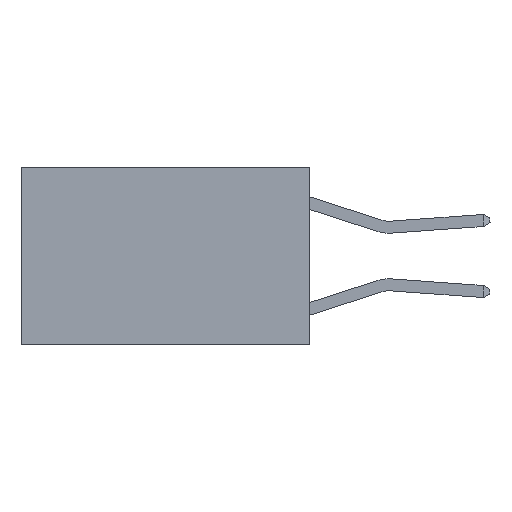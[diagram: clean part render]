
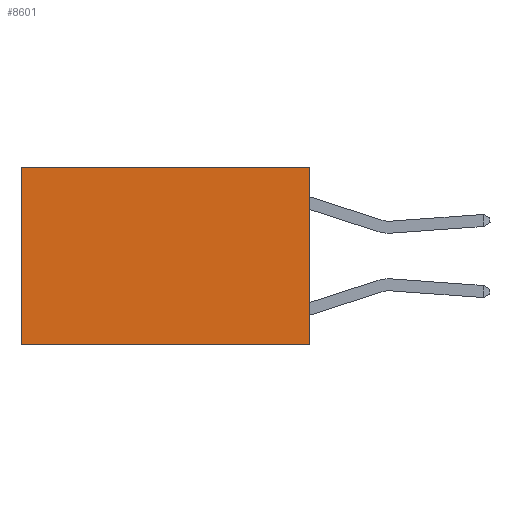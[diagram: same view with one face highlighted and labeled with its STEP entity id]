
A CAD part, left-side view. The second image highlights one B-rep face of the part: STEP entity #8601.
In plain terms, the highlighted planar face has unit normal (-1, 0, 0).
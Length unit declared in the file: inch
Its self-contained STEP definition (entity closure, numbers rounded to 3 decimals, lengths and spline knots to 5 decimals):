
#12 = AXIS2_PLACEMENT_3D ( 'NONE', #1981, #5078, #3626 ) ;
#113 = VERTEX_POINT ( 'NONE', #5423 ) ;
#270 = LINE ( 'NONE', #6332, #7878 ) ;
#493 = DIRECTION ( 'NONE',  ( 0., 0., -1. ) ) ;
#981 = CARTESIAN_POINT ( 'NONE',  ( 0.2625, 0.6, 0. ) ) ;
#1028 = VERTEX_POINT ( 'NONE', #8412 ) ;
#1563 = ORIENTED_EDGE ( 'NONE', *, *, #1692, .T. ) ;
#1692 = EDGE_CURVE ( 'NONE', #1028, #9259, #5855, .T. ) ;
#1696 = ORIENTED_EDGE ( 'NONE', *, *, #2948, .F. ) ;
#1785 = ORIENTED_EDGE ( 'NONE', *, *, #6301, .F. ) ;
#1795 = ORIENTED_EDGE ( 'NONE', *, *, #7056, .T. ) ;
#1848 = DIRECTION ( 'NONE',  ( 0., 0., -1. ) ) ;
#1981 = CARTESIAN_POINT ( 'NONE',  ( 0.2625, 0., 0. ) ) ;
#2857 = PLANE ( 'NONE',  #12 ) ;
#2948 = EDGE_CURVE ( 'NONE', #1028, #113, #7876, .T. ) ;
#3189 = DIRECTION ( 'NONE',  ( 0., 1., 0. ) ) ;
#3626 = DIRECTION ( 'NONE',  ( 0., 0., -1. ) ) ;
#4544 = LINE ( 'NONE', #4900, #5945 ) ;
#4815 = FACE_OUTER_BOUND ( 'NONE', #6292, .T. ) ;
#4900 = CARTESIAN_POINT ( 'NONE',  ( 0.2625, 0., -0.37 ) ) ;
#5078 = DIRECTION ( 'NONE',  ( 1., 0., 0. ) ) ;
#5423 = CARTESIAN_POINT ( 'NONE',  ( 0.2625, 0., -0.37 ) ) ;
#5486 = CARTESIAN_POINT ( 'NONE',  ( 0.2625, 0.6, -0.37 ) ) ;
#5645 = VECTOR ( 'NONE', #3189, 39.37008 ) ;
#5822 = CARTESIAN_POINT ( 'NONE',  ( 0.2625, 0., 0. ) ) ;
#5855 = LINE ( 'NONE', #8442, #5645 ) ;
#5945 = VECTOR ( 'NONE', #9075, 39.37008 ) ;
#6292 = EDGE_LOOP ( 'NONE', ( #1795, #1785, #1696, #1563 ) ) ;
#6301 = EDGE_CURVE ( 'NONE', #113, #7470, #4544, .T. ) ;
#6332 = CARTESIAN_POINT ( 'NONE',  ( 0.2625, 0.6, 0. ) ) ;
#7056 = EDGE_CURVE ( 'NONE', #9259, #7470, #270, .T. ) ;
#7470 = VERTEX_POINT ( 'NONE', #5486 ) ;
#7876 = LINE ( 'NONE', #5822, #8078 ) ;
#7878 = VECTOR ( 'NONE', #1848, 39.37008 ) ;
#8078 = VECTOR ( 'NONE', #493, 39.37008 ) ;
#8412 = CARTESIAN_POINT ( 'NONE',  ( 0.2625, 0., 0. ) ) ;
#8442 = CARTESIAN_POINT ( 'NONE',  ( 0.2625, 0., 0. ) ) ;
#8601 = ADVANCED_FACE ( 'NONE', ( #4815 ), #2857, .F. ) ;
#9075 = DIRECTION ( 'NONE',  ( 0., 1., 0. ) ) ;
#9259 = VERTEX_POINT ( 'NONE', #981 ) ;
